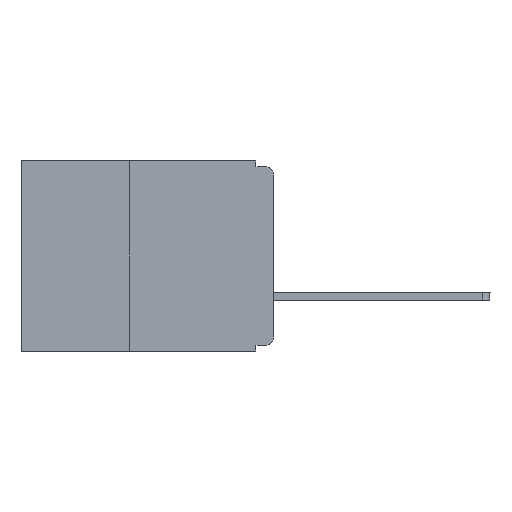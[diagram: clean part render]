
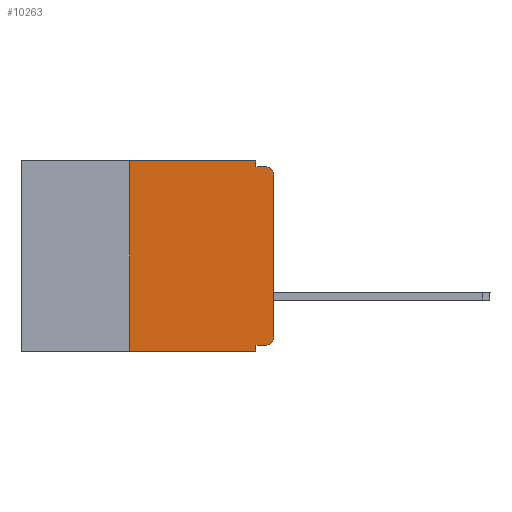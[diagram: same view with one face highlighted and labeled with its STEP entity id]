
A CAD part, left-side view. The second image highlights one B-rep face of the part: STEP entity #10263.
In plain terms, the highlighted planar face has unit normal (-1, 0, 0).
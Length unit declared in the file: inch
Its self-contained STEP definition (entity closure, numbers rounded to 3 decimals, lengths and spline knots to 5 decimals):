
#139 = VERTEX_POINT ( 'NONE', #1812 ) ;
#543 = CARTESIAN_POINT ( 'NONE',  ( 0., 0.015, -0.025 ) ) ;
#654 = CARTESIAN_POINT ( 'NONE',  ( 0., 0.031, 0. ) ) ;
#683 = DIRECTION ( 'NONE',  ( 0., 0., -1. ) ) ;
#1020 = CARTESIAN_POINT ( 'NONE',  ( 0., 0.25, -0.33 ) ) ;
#1038 = EDGE_CURVE ( 'NONE', #139, #13598, #11253, .T. ) ;
#1236 = CARTESIAN_POINT ( 'NONE',  ( 0., 0., -0.32 ) ) ;
#1273 = LINE ( 'NONE', #3651, #11890 ) ;
#1400 = CIRCLE ( 'NONE', #13000, 0.015 ) ;
#1428 = FACE_OUTER_BOUND ( 'NONE', #13446, .T. ) ;
#1812 = CARTESIAN_POINT ( 'NONE',  ( 0., 0.25, 0. ) ) ;
#1869 = CARTESIAN_POINT ( 'NONE',  ( 0., 0.437, 0. ) ) ;
#1916 = CARTESIAN_POINT ( 'NONE',  ( 0., 0.031, -0.33 ) ) ;
#2177 = DIRECTION ( 'NONE',  ( 0., -1., 0. ) ) ;
#2213 = ORIENTED_EDGE ( 'NONE', *, *, #6242, .T. ) ;
#2538 = VERTEX_POINT ( 'NONE', #4907 ) ;
#3125 = DIRECTION ( 'NONE',  ( 0., -1., 0. ) ) ;
#3170 = CARTESIAN_POINT ( 'NONE',  ( 0., 0., -0.025 ) ) ;
#3171 = CARTESIAN_POINT ( 'NONE',  ( 0., 0.25, -0.33 ) ) ;
#3651 = CARTESIAN_POINT ( 'NONE',  ( 0., 0., 0. ) ) ;
#3822 = PLANE ( 'NONE',  #5055 ) ;
#4000 = ORIENTED_EDGE ( 'NONE', *, *, #15382, .F. ) ;
#4400 = EDGE_CURVE ( 'NONE', #6541, #6556, #1273, .T. ) ;
#4655 = VECTOR ( 'NONE', #3125, 39.37008 ) ;
#4700 = VERTEX_POINT ( 'NONE', #3171 ) ;
#4802 = VERTEX_POINT ( 'NONE', #7044 ) ;
#4823 = VECTOR ( 'NONE', #2177, 39.37008 ) ;
#4894 = DIRECTION ( 'NONE',  ( 0., 0., -1. ) ) ;
#4907 = CARTESIAN_POINT ( 'NONE',  ( 0., 0.031, -0.01 ) ) ;
#5055 = AXIS2_PLACEMENT_3D ( 'NONE', #8602, #6310, #14869 ) ;
#5254 = ORIENTED_EDGE ( 'NONE', *, *, #6550, .F. ) ;
#5550 = DIRECTION ( 'NONE',  ( -1., 0., 0. ) ) ;
#6001 = LINE ( 'NONE', #12017, #4823 ) ;
#6180 = ORIENTED_EDGE ( 'NONE', *, *, #4400, .T. ) ;
#6242 = EDGE_CURVE ( 'NONE', #6556, #10506, #1400, .T. ) ;
#6310 = DIRECTION ( 'NONE',  ( 1., 0., 0. ) ) ;
#6398 = LINE ( 'NONE', #1916, #12805 ) ;
#6533 = VERTEX_POINT ( 'NONE', #12964 ) ;
#6541 = VERTEX_POINT ( 'NONE', #10999 ) ;
#6550 = EDGE_CURVE ( 'NONE', #6533, #11778, #6398, .T. ) ;
#6556 = VERTEX_POINT ( 'NONE', #3170 ) ;
#7044 = CARTESIAN_POINT ( 'NONE',  ( 0., 0.015, -0.32 ) ) ;
#7239 = ORIENTED_EDGE ( 'NONE', *, *, #15714, .T. ) ;
#7424 = ORIENTED_EDGE ( 'NONE', *, *, #1038, .F. ) ;
#7458 = EDGE_CURVE ( 'NONE', #4700, #11778, #9271, .T. ) ;
#7670 = DIRECTION ( 'NONE',  ( 0., -1., 0. ) ) ;
#8602 = CARTESIAN_POINT ( 'NONE',  ( 0., 0.437, 0. ) ) ;
#8705 = LINE ( 'NONE', #1020, #15670 ) ;
#8787 = DIRECTION ( 'NONE',  ( 0., 0., -1. ) ) ;
#8801 = VECTOR ( 'NONE', #9874, 39.37008 ) ;
#8895 = VECTOR ( 'NONE', #7670, 39.37008 ) ;
#9080 = AXIS2_PLACEMENT_3D ( 'NONE', #14645, #11125, #4894 ) ;
#9271 = LINE ( 'NONE', #15027, #8895 ) ;
#9585 = EDGE_CURVE ( 'NONE', #4802, #6533, #13233, .T. ) ;
#9642 = DIRECTION ( 'NONE',  ( 0., 0., 1. ) ) ;
#9874 = DIRECTION ( 'NONE',  ( 0., 1., 0. ) ) ;
#9934 = EDGE_CURVE ( 'NONE', #13598, #2538, #11290, .T. ) ;
#10047 = DIRECTION ( 'NONE',  ( 0., 0., 1. ) ) ;
#10081 = CARTESIAN_POINT ( 'NONE',  ( 0., 0.031, 0. ) ) ;
#10263 = ADVANCED_FACE ( 'NONE', ( #1428 ), #3822, .F. ) ;
#10437 = CARTESIAN_POINT ( 'NONE',  ( 0., 0.031, -0.33 ) ) ;
#10506 = VERTEX_POINT ( 'NONE', #15889 ) ;
#10634 = DIRECTION ( 'NONE',  ( 0., 0., -1. ) ) ;
#10797 = ORIENTED_EDGE ( 'NONE', *, *, #14713, .F. ) ;
#10999 = CARTESIAN_POINT ( 'NONE',  ( 0., 0., -0.305 ) ) ;
#11008 = ORIENTED_EDGE ( 'NONE', *, *, #9585, .F. ) ;
#11125 = DIRECTION ( 'NONE',  ( -1., 0., 0. ) ) ;
#11253 = LINE ( 'NONE', #1869, #4655 ) ;
#11290 = LINE ( 'NONE', #10081, #13993 ) ;
#11778 = VERTEX_POINT ( 'NONE', #10437 ) ;
#11890 = VECTOR ( 'NONE', #10047, 39.37008 ) ;
#12017 = CARTESIAN_POINT ( 'NONE',  ( 0., 0., -0.01 ) ) ;
#12550 = CIRCLE ( 'NONE', #9080, 0.015 ) ;
#12805 = VECTOR ( 'NONE', #683, 39.37008 ) ;
#12964 = CARTESIAN_POINT ( 'NONE',  ( 0., 0.031, -0.32 ) ) ;
#13000 = AXIS2_PLACEMENT_3D ( 'NONE', #543, #5550, #10634 ) ;
#13233 = LINE ( 'NONE', #1236, #8801 ) ;
#13446 = EDGE_LOOP ( 'NONE', ( #6180, #2213, #10797, #15068, #7424, #4000, #15896, #5254, #11008, #7239 ) ) ;
#13598 = VERTEX_POINT ( 'NONE', #654 ) ;
#13993 = VECTOR ( 'NONE', #8787, 39.37008 ) ;
#14645 = CARTESIAN_POINT ( 'NONE',  ( 0., 0.015, -0.305 ) ) ;
#14713 = EDGE_CURVE ( 'NONE', #2538, #10506, #6001, .T. ) ;
#14869 = DIRECTION ( 'NONE',  ( 0., 0., -1. ) ) ;
#15027 = CARTESIAN_POINT ( 'NONE',  ( 0., 0.437, -0.33 ) ) ;
#15068 = ORIENTED_EDGE ( 'NONE', *, *, #9934, .F. ) ;
#15382 = EDGE_CURVE ( 'NONE', #4700, #139, #8705, .T. ) ;
#15670 = VECTOR ( 'NONE', #9642, 39.37008 ) ;
#15714 = EDGE_CURVE ( 'NONE', #4802, #6541, #12550, .T. ) ;
#15889 = CARTESIAN_POINT ( 'NONE',  ( 0., 0.015, -0.01 ) ) ;
#15896 = ORIENTED_EDGE ( 'NONE', *, *, #7458, .T. ) ;
